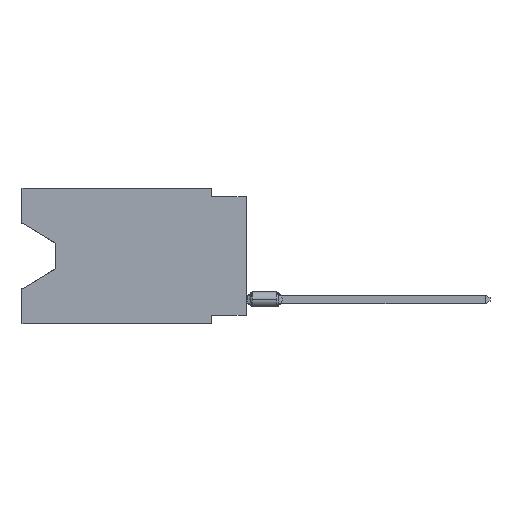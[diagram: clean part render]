
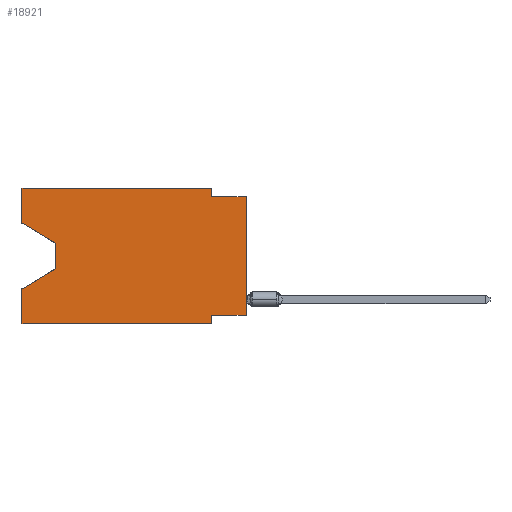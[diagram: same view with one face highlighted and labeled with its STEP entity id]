
A CAD part, left-side view. The second image highlights one B-rep face of the part: STEP entity #18921.
In plain terms, the highlighted planar face has unit normal (-1, 0, 0).
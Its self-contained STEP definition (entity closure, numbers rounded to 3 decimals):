
#58 = VERTEX_POINT ( 'NONE', #11572 ) ;
#1055 = EDGE_CURVE ( 'NONE', #16277, #1484, #29627, .T. ) ;
#1484 = VERTEX_POINT ( 'NONE', #35460 ) ;
#2230 = ORIENTED_EDGE ( 'NONE', *, *, #28861, .T. ) ;
#2309 = CARTESIAN_POINT ( 'NONE',  ( 0., 16.383, 0. ) ) ;
#2810 = DIRECTION ( 'NONE',  ( 0., 0., -1. ) ) ;
#2835 = VECTOR ( 'NONE', #29337, 1000. ) ;
#3067 = VERTEX_POINT ( 'NONE', #25031 ) ;
#3235 = ORIENTED_EDGE ( 'NONE', *, *, #35579, .F. ) ;
#3274 = VERTEX_POINT ( 'NONE', #11764 ) ;
#3831 = VECTOR ( 'NONE', #2810, 1000. ) ;
#3967 = CARTESIAN_POINT ( 'NONE',  ( 0., 13.97, -5.893 ) ) ;
#4036 = DIRECTION ( 'NONE',  ( 1., 0., 0. ) ) ;
#5081 = CARTESIAN_POINT ( 'NONE',  ( 0., 13.97, -4.013 ) ) ;
#5725 = DIRECTION ( 'NONE',  ( 0., -1., 0. ) ) ;
#6636 = ORIENTED_EDGE ( 'NONE', *, *, #21707, .T. ) ;
#6913 = ORIENTED_EDGE ( 'NONE', *, *, #20691, .F. ) ;
#6960 = CARTESIAN_POINT ( 'NONE',  ( 0., 16.383, 0. ) ) ;
#7184 = AXIS2_PLACEMENT_3D ( 'NONE', #27518, #4036, #30196 ) ;
#7310 = ORIENTED_EDGE ( 'NONE', *, *, #26724, .F. ) ;
#7441 = PLANE ( 'NONE',  #7184 ) ;
#7548 = ORIENTED_EDGE ( 'NONE', *, *, #34691, .F. ) ;
#9391 = CARTESIAN_POINT ( 'NONE',  ( 0., 16.383, 0. ) ) ;
#9534 = DIRECTION ( 'NONE',  ( 0., 1., 0. ) ) ;
#9647 = DIRECTION ( 'NONE',  ( 0., -1., 0. ) ) ;
#9877 = ORIENTED_EDGE ( 'NONE', *, *, #21726, .T. ) ;
#10000 = CARTESIAN_POINT ( 'NONE',  ( 0., 13.97, -4.013 ) ) ;
#10914 = ORIENTED_EDGE ( 'NONE', *, *, #34354, .T. ) ;
#11331 = LINE ( 'NONE', #11715, #17275 ) ;
#11572 = CARTESIAN_POINT ( 'NONE',  ( 0., 2.54, -9.906 ) ) ;
#11715 = CARTESIAN_POINT ( 'NONE',  ( 0., 0., -0.635 ) ) ;
#11764 = CARTESIAN_POINT ( 'NONE',  ( 0., 13.97, -5.893 ) ) ;
#11796 = VECTOR ( 'NONE', #21042, 1000. ) ;
#12017 = VERTEX_POINT ( 'NONE', #16604 ) ;
#13047 = CARTESIAN_POINT ( 'NONE',  ( 0., 16.383, 0. ) ) ;
#13536 = CARTESIAN_POINT ( 'NONE',  ( 0., 16.383, -9.906 ) ) ;
#15265 = DIRECTION ( 'NONE',  ( 0., 0., 1. ) ) ;
#15475 = VECTOR ( 'NONE', #15265, 1000. ) ;
#15922 = CARTESIAN_POINT ( 'NONE',  ( 0., 0., -9.271 ) ) ;
#16277 = VERTEX_POINT ( 'NONE', #15922 ) ;
#16604 = CARTESIAN_POINT ( 'NONE',  ( 0., 16.383, -7.36 ) ) ;
#16637 = LINE ( 'NONE', #28386, #37091 ) ;
#17201 = LINE ( 'NONE', #5081, #3831 ) ;
#17217 = VECTOR ( 'NONE', #9647, 1000. ) ;
#17275 = VECTOR ( 'NONE', #19664, 1000. ) ;
#17609 = DIRECTION ( 'NONE',  ( 0., 0.855, -0.519 ) ) ;
#18390 = LINE ( 'NONE', #29578, #11796 ) ;
#18730 = VECTOR ( 'NONE', #5725, 1000. ) ;
#18921 = ADVANCED_FACE ( 'NONE', ( #36238 ), #7441, .F. ) ;
#19136 = CARTESIAN_POINT ( 'NONE',  ( 0., 16.383, -2.546 ) ) ;
#19641 = VERTEX_POINT ( 'NONE', #21369 ) ;
#19664 = DIRECTION ( 'NONE',  ( 0., -1., 0. ) ) ;
#19722 = VERTEX_POINT ( 'NONE', #10000 ) ;
#19874 = VERTEX_POINT ( 'NONE', #23942 ) ;
#19901 = CARTESIAN_POINT ( 'NONE',  ( 0., 0., 0. ) ) ;
#20000 = VECTOR ( 'NONE', #9534, 1000. ) ;
#20691 = EDGE_CURVE ( 'NONE', #19874, #3067, #35219, .T. ) ;
#21042 = DIRECTION ( 'NONE',  ( 0., 0., -1. ) ) ;
#21369 = CARTESIAN_POINT ( 'NONE',  ( 0., 16.383, -9.906 ) ) ;
#21707 = EDGE_CURVE ( 'NONE', #19722, #3274, #17201, .T. ) ;
#21726 = EDGE_CURVE ( 'NONE', #33133, #19722, #16637, .T. ) ;
#23114 = DIRECTION ( 'NONE',  ( 0., 0., 1. ) ) ;
#23942 = CARTESIAN_POINT ( 'NONE',  ( 0., 2.54, 0. ) ) ;
#24909 = EDGE_LOOP ( 'NONE', ( #9877, #6636, #2230, #34732, #36525, #3235, #36229, #10914, #7548, #6913, #7310, #36420 ) ) ;
#24916 = LINE ( 'NONE', #13536, #17217 ) ;
#24964 = VERTEX_POINT ( 'NONE', #13047 ) ;
#25031 = CARTESIAN_POINT ( 'NONE',  ( 0., 2.54, -0.635 ) ) ;
#25928 = DIRECTION ( 'NONE',  ( 0., -0.855, -0.519 ) ) ;
#26724 = EDGE_CURVE ( 'NONE', #24964, #19874, #36995, .T. ) ;
#27038 = LINE ( 'NONE', #6960, #36217 ) ;
#27518 = CARTESIAN_POINT ( 'NONE',  ( 0., 16.383, 0. ) ) ;
#27712 = EDGE_CURVE ( 'NONE', #19641, #12017, #27038, .T. ) ;
#28386 = CARTESIAN_POINT ( 'NONE',  ( 0., 16.383, -2.546 ) ) ;
#28861 = EDGE_CURVE ( 'NONE', #3274, #12017, #29932, .T. ) ;
#29337 = DIRECTION ( 'NONE',  ( 0., 0., -1. ) ) ;
#29578 = CARTESIAN_POINT ( 'NONE',  ( 0., 2.54, -9.906 ) ) ;
#29627 = LINE ( 'NONE', #35500, #20000 ) ;
#29897 = DIRECTION ( 'NONE',  ( 0., 0., 1. ) ) ;
#29932 = LINE ( 'NONE', #3967, #32678 ) ;
#30196 = DIRECTION ( 'NONE',  ( 0., 0., -1. ) ) ;
#31290 = LINE ( 'NONE', #19901, #34816 ) ;
#31631 = CARTESIAN_POINT ( 'NONE',  ( 0., 2.54, 0. ) ) ;
#32678 = VECTOR ( 'NONE', #17609, 1000. ) ;
#33133 = VERTEX_POINT ( 'NONE', #19136 ) ;
#33276 = VERTEX_POINT ( 'NONE', #36567 ) ;
#33504 = EDGE_CURVE ( 'NONE', #19641, #58, #24916, .T. ) ;
#34354 = EDGE_CURVE ( 'NONE', #16277, #33276, #31290, .T. ) ;
#34691 = EDGE_CURVE ( 'NONE', #3067, #33276, #11331, .T. ) ;
#34732 = ORIENTED_EDGE ( 'NONE', *, *, #27712, .F. ) ;
#34816 = VECTOR ( 'NONE', #23114, 1000. ) ;
#35219 = LINE ( 'NONE', #31631, #2835 ) ;
#35364 = LINE ( 'NONE', #9391, #15475 ) ;
#35460 = CARTESIAN_POINT ( 'NONE',  ( 0., 2.54, -9.271 ) ) ;
#35500 = CARTESIAN_POINT ( 'NONE',  ( 0., 0., -9.271 ) ) ;
#35579 = EDGE_CURVE ( 'NONE', #1484, #58, #18390, .T. ) ;
#36217 = VECTOR ( 'NONE', #29897, 1000. ) ;
#36229 = ORIENTED_EDGE ( 'NONE', *, *, #1055, .F. ) ;
#36238 = FACE_OUTER_BOUND ( 'NONE', #24909, .T. ) ;
#36420 = ORIENTED_EDGE ( 'NONE', *, *, #36481, .F. ) ;
#36481 = EDGE_CURVE ( 'NONE', #33133, #24964, #35364, .T. ) ;
#36525 = ORIENTED_EDGE ( 'NONE', *, *, #33504, .T. ) ;
#36567 = CARTESIAN_POINT ( 'NONE',  ( 0., 0., -0.635 ) ) ;
#36995 = LINE ( 'NONE', #2309, #18730 ) ;
#37091 = VECTOR ( 'NONE', #25928, 1000. ) ;
